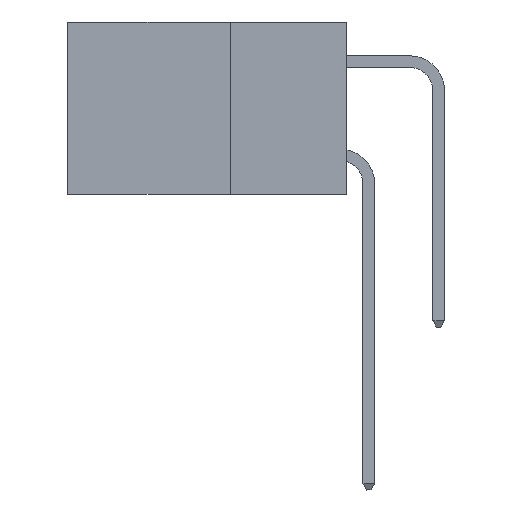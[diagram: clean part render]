
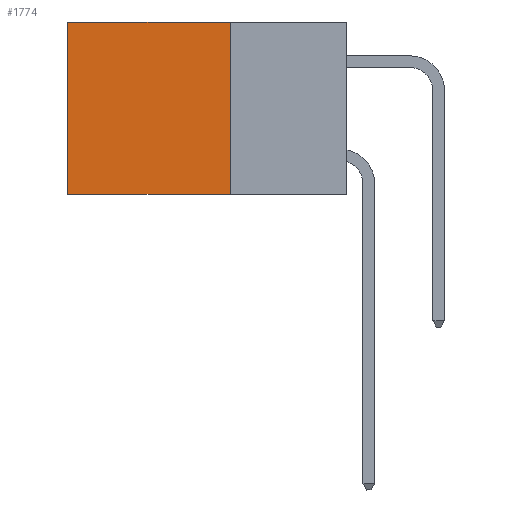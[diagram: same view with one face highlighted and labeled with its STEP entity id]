
A CAD part, left-side view. The second image highlights one B-rep face of the part: STEP entity #1774.
In plain terms, the highlighted planar face has unit normal (-1, 0, 0).
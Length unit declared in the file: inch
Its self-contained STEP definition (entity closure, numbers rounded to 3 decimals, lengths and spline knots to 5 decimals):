
#1421 = EDGE_LOOP ( 'NONE', ( #17674, #6629, #4797, #15210 ) ) ;
#1620 = VERTEX_POINT ( 'NONE', #3742 ) ;
#1774 = ADVANCED_FACE ( 'NONE', ( #19777 ), #10620, .F. ) ;
#2058 = EDGE_CURVE ( 'NONE', #22904, #20204, #13351, .T. ) ;
#3742 = CARTESIAN_POINT ( 'NONE',  ( 0.2875, 0.25, 0. ) ) ;
#4330 = CARTESIAN_POINT ( 'NONE',  ( 0.2875, 0.6, -0.37 ) ) ;
#4797 = ORIENTED_EDGE ( 'NONE', *, *, #6671, .F. ) ;
#4832 = LINE ( 'NONE', #10865, #20462 ) ;
#5471 = CARTESIAN_POINT ( 'NONE',  ( 0.2875, 0.25, 0. ) ) ;
#6629 = ORIENTED_EDGE ( 'NONE', *, *, #2058, .F. ) ;
#6671 = EDGE_CURVE ( 'NONE', #1620, #22904, #21051, .T. ) ;
#8102 = CARTESIAN_POINT ( 'NONE',  ( 0.2875, 0.25, 0. ) ) ;
#8666 = DIRECTION ( 'NONE',  ( 0., 0., -1. ) ) ;
#9544 = LINE ( 'NONE', #5471, #10984 ) ;
#10620 = PLANE ( 'NONE',  #29152 ) ;
#10865 = CARTESIAN_POINT ( 'NONE',  ( 0.2875, 0.6, 0. ) ) ;
#10984 = VECTOR ( 'NONE', #28074, 39.37008 ) ;
#11111 = DIRECTION ( 'NONE',  ( 0., 0., -1. ) ) ;
#11201 = EDGE_CURVE ( 'NONE', #19608, #20204, #4832, .T. ) ;
#13351 = LINE ( 'NONE', #21041, #15842 ) ;
#14711 = CARTESIAN_POINT ( 'NONE',  ( 0.2875, 0.25, -0.37 ) ) ;
#14792 = DIRECTION ( 'NONE',  ( 0., 0., -1. ) ) ;
#15210 = ORIENTED_EDGE ( 'NONE', *, *, #21786, .T. ) ;
#15842 = VECTOR ( 'NONE', #25491, 39.37008 ) ;
#17674 = ORIENTED_EDGE ( 'NONE', *, *, #11201, .T. ) ;
#19608 = VERTEX_POINT ( 'NONE', #24708 ) ;
#19777 = FACE_OUTER_BOUND ( 'NONE', #1421, .T. ) ;
#20204 = VERTEX_POINT ( 'NONE', #4330 ) ;
#20273 = DIRECTION ( 'NONE',  ( 1., 0., 0. ) ) ;
#20462 = VECTOR ( 'NONE', #8666, 39.37008 ) ;
#21041 = CARTESIAN_POINT ( 'NONE',  ( 0.2875, 0.25, -0.37 ) ) ;
#21051 = LINE ( 'NONE', #8102, #27073 ) ;
#21786 = EDGE_CURVE ( 'NONE', #1620, #19608, #9544, .T. ) ;
#22904 = VERTEX_POINT ( 'NONE', #14711 ) ;
#24708 = CARTESIAN_POINT ( 'NONE',  ( 0.2875, 0.6, 0. ) ) ;
#25491 = DIRECTION ( 'NONE',  ( 0., 1., 0. ) ) ;
#26505 = CARTESIAN_POINT ( 'NONE',  ( 0.2875, 0.25, 0. ) ) ;
#27073 = VECTOR ( 'NONE', #14792, 39.37008 ) ;
#28074 = DIRECTION ( 'NONE',  ( 0., 1., 0. ) ) ;
#29152 = AXIS2_PLACEMENT_3D ( 'NONE', #26505, #20273, #11111 ) ;
